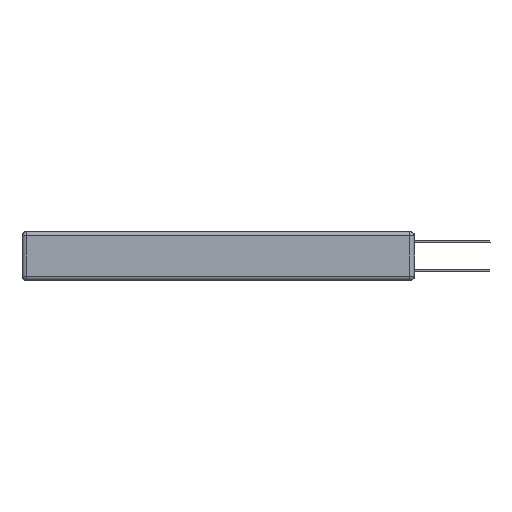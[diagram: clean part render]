
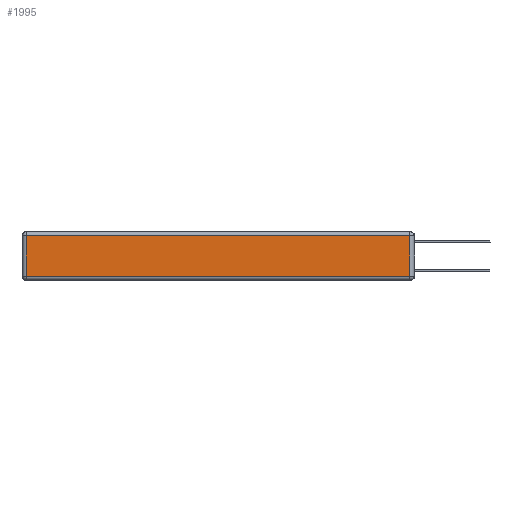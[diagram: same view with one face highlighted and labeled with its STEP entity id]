
A CAD part, left-side view. The second image highlights one B-rep face of the part: STEP entity #1995.
In plain terms, the highlighted planar face has unit normal (-1, 0, 0).
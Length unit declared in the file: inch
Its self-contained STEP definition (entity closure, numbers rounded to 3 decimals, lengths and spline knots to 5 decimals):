
#860 = EDGE_LOOP ( 'NONE', ( #1676, #20795, #13690, #2206 ) ) ;
#1602 = DIRECTION ( 'NONE',  ( 0., 0., -1. ) ) ;
#1676 = ORIENTED_EDGE ( 'NONE', *, *, #6459, .T. ) ;
#1995 = ADVANCED_FACE ( 'NONE', ( #8354 ), #21024, .T. ) ;
#2206 = ORIENTED_EDGE ( 'NONE', *, *, #21049, .T. ) ;
#2848 = CARTESIAN_POINT ( 'NONE',  ( 0., 0., -0.313 ) ) ;
#4145 = CARTESIAN_POINT ( 'NONE',  ( 0., 2.75, -0.03 ) ) ;
#5421 = AXIS2_PLACEMENT_3D ( 'NONE', #20932, #17106, #12573 ) ;
#6036 = VECTOR ( 'NONE', #11345, 39.37008 ) ;
#6459 = EDGE_CURVE ( 'NONE', #23880, #23614, #26243, .T. ) ;
#6852 = VECTOR ( 'NONE', #20592, 39.37008 ) ;
#8354 = FACE_OUTER_BOUND ( 'NONE', #860, .T. ) ;
#10733 = LINE ( 'NONE', #24552, #11400 ) ;
#11345 = DIRECTION ( 'NONE',  ( 0., 0., 1. ) ) ;
#11400 = VECTOR ( 'NONE', #1602, 39.37008 ) ;
#11467 = DIRECTION ( 'NONE',  ( 0., -1., 0. ) ) ;
#12573 = DIRECTION ( 'NONE',  ( 0., 0., 1. ) ) ;
#13690 = ORIENTED_EDGE ( 'NONE', *, *, #17639, .T. ) ;
#14295 = CARTESIAN_POINT ( 'NONE',  ( 0., 2.72, -0.313 ) ) ;
#14823 = EDGE_CURVE ( 'NONE', #23614, #17001, #15161, .T. ) ;
#15161 = LINE ( 'NONE', #23747, #6036 ) ;
#17001 = VERTEX_POINT ( 'NONE', #20722 ) ;
#17106 = DIRECTION ( 'NONE',  ( -1., 0., 0. ) ) ;
#17639 = EDGE_CURVE ( 'NONE', #17001, #24118, #17936, .T. ) ;
#17936 = LINE ( 'NONE', #4145, #6852 ) ;
#19064 = VECTOR ( 'NONE', #11467, 39.37008 ) ;
#20592 = DIRECTION ( 'NONE',  ( 0., 1., 0. ) ) ;
#20722 = CARTESIAN_POINT ( 'NONE',  ( 0., 0.03, -0.03 ) ) ;
#20795 = ORIENTED_EDGE ( 'NONE', *, *, #14823, .T. ) ;
#20932 = CARTESIAN_POINT ( 'NONE',  ( 0., 0., -0.343 ) ) ;
#21024 = PLANE ( 'NONE',  #5421 ) ;
#21049 = EDGE_CURVE ( 'NONE', #24118, #23880, #10733, .T. ) ;
#21543 = CARTESIAN_POINT ( 'NONE',  ( 0., 2.72, -0.03 ) ) ;
#23614 = VERTEX_POINT ( 'NONE', #24127 ) ;
#23747 = CARTESIAN_POINT ( 'NONE',  ( 0., 0.03, -0.343 ) ) ;
#23880 = VERTEX_POINT ( 'NONE', #14295 ) ;
#24118 = VERTEX_POINT ( 'NONE', #21543 ) ;
#24127 = CARTESIAN_POINT ( 'NONE',  ( 0., 0.03, -0.313 ) ) ;
#24552 = CARTESIAN_POINT ( 'NONE',  ( 0., 2.72, -0.343 ) ) ;
#26243 = LINE ( 'NONE', #2848, #19064 ) ;
